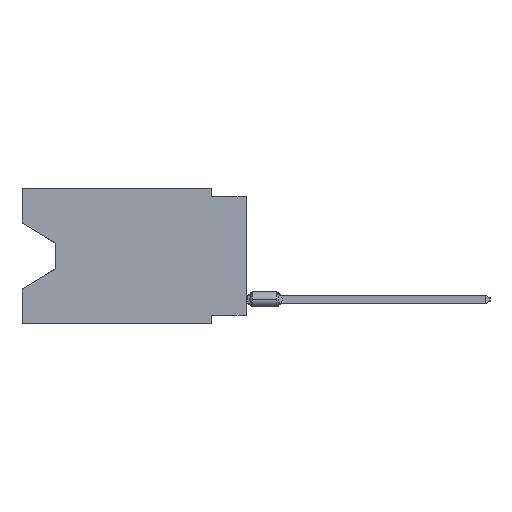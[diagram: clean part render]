
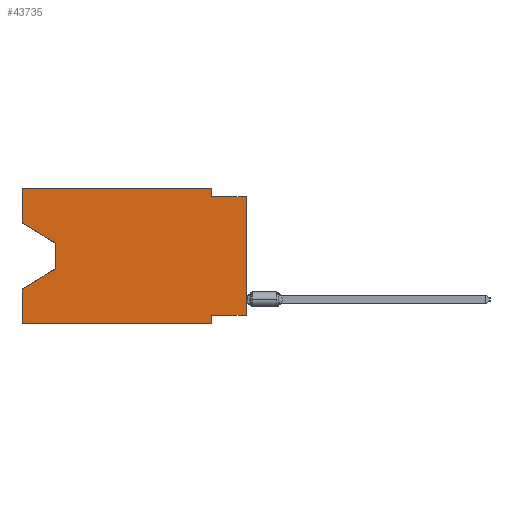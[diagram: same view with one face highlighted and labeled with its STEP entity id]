
A CAD part, left-side view. The second image highlights one B-rep face of the part: STEP entity #43735.
In plain terms, the highlighted planar face has unit normal (-1, 0, 0).
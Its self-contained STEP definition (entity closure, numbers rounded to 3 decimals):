
#249 = DIRECTION ( 'NONE',  ( 0., 0., 1. ) ) ;
#248 = VECTOR ( 'NONE', #21182, 1000. ) ;
#1300 = LINE ( 'NONE', #32505, #5962 ) ;
#2543 = LINE ( 'NONE', #37479, #35545 ) ;
#2876 = EDGE_CURVE ( 'NONE', #18927, #43641, #38914, .T. ) ;
#3427 = CARTESIAN_POINT ( 'NONE',  ( 0., 16.383, 0. ) ) ;
#4253 = VERTEX_POINT ( 'NONE', #3427 ) ;
#4367 = DIRECTION ( 'NONE',  ( 0., -1., 0. ) ) ;
#4447 = AXIS2_PLACEMENT_3D ( 'NONE', #50003, #10769, #25622 ) ;
#4461 = EDGE_CURVE ( 'NONE', #8686, #4253, #44630, .T. ) ;
#4482 = VERTEX_POINT ( 'NONE', #36317 ) ;
#5019 = ORIENTED_EDGE ( 'NONE', *, *, #14793, .F. ) ;
#5115 = CARTESIAN_POINT ( 'NONE',  ( 0., 0., 0. ) ) ;
#5689 = DIRECTION ( 'NONE',  ( 0., 0., 1. ) ) ;
#5962 = VECTOR ( 'NONE', #36523, 1000. ) ;
#7322 = DIRECTION ( 'NONE',  ( 0., 1., 0. ) ) ;
#8686 = VERTEX_POINT ( 'NONE', #26332 ) ;
#10237 = CARTESIAN_POINT ( 'NONE',  ( 0., 16.383, 0. ) ) ;
#10769 = DIRECTION ( 'NONE',  ( 1., 0., 0. ) ) ;
#11492 = EDGE_CURVE ( 'NONE', #17639, #19526, #2543, .T. ) ;
#11614 = LINE ( 'NONE', #29082, #48688 ) ;
#12200 = ORIENTED_EDGE ( 'NONE', *, *, #42566, .T. ) ;
#12966 = LINE ( 'NONE', #17823, #46207 ) ;
#13484 = EDGE_CURVE ( 'NONE', #18006, #26070, #25495, .T. ) ;
#13717 = CARTESIAN_POINT ( 'NONE',  ( 0., 16.383, 0. ) ) ;
#14038 = VECTOR ( 'NONE', #16965, 1000. ) ;
#14118 = EDGE_CURVE ( 'NONE', #42230, #4482, #30687, .T. ) ;
#14709 = CARTESIAN_POINT ( 'NONE',  ( 0., 13.97, -4.013 ) ) ;
#14792 = VECTOR ( 'NONE', #249, 1000. ) ;
#14793 = EDGE_CURVE ( 'NONE', #36934, #18006, #11614, .T. ) ;
#15066 = PLANE ( 'NONE',  #4447 ) ;
#15119 = DIRECTION ( 'NONE',  ( 0., 0., -1. ) ) ;
#15991 = DIRECTION ( 'NONE',  ( 0., -1., 0. ) ) ;
#16433 = CARTESIAN_POINT ( 'NONE',  ( 0., 16.383, -2.546 ) ) ;
#16965 = DIRECTION ( 'NONE',  ( 0., 0., -1. ) ) ;
#17252 = VECTOR ( 'NONE', #22578, 1000. ) ;
#17639 = VERTEX_POINT ( 'NONE', #36337 ) ;
#17823 = CARTESIAN_POINT ( 'NONE',  ( 0., 16.383, -9.906 ) ) ;
#18006 = VERTEX_POINT ( 'NONE', #36483 ) ;
#18927 = VERTEX_POINT ( 'NONE', #47924 ) ;
#19526 = VERTEX_POINT ( 'NONE', #38379 ) ;
#21182 = DIRECTION ( 'NONE',  ( 0., 0., -1. ) ) ;
#22578 = DIRECTION ( 'NONE',  ( 0., 0., 1. ) ) ;
#22694 = ORIENTED_EDGE ( 'NONE', *, *, #50847, .F. ) ;
#24102 = ORIENTED_EDGE ( 'NONE', *, *, #52577, .T. ) ;
#24240 = EDGE_LOOP ( 'NONE', ( #31747, #39656, #24102, #39378, #37430, #52296, #5019, #12200, #46076, #22694, #45834, #32801 ) ) ;
#24972 = VECTOR ( 'NONE', #33895, 1000. ) ;
#25495 = LINE ( 'NONE', #42964, #248 ) ;
#25622 = DIRECTION ( 'NONE',  ( 0., 0., -1. ) ) ;
#26070 = VERTEX_POINT ( 'NONE', #55886 ) ;
#26332 = CARTESIAN_POINT ( 'NONE',  ( 0., 16.383, -2.546 ) ) ;
#26478 = EDGE_CURVE ( 'NONE', #18927, #26070, #12966, .T. ) ;
#27667 = CARTESIAN_POINT ( 'NONE',  ( 0., 16.383, -7.36 ) ) ;
#28839 = LINE ( 'NONE', #36872, #29584 ) ;
#29082 = CARTESIAN_POINT ( 'NONE',  ( 0., 0., -9.271 ) ) ;
#29584 = VECTOR ( 'NONE', #15119, 1000. ) ;
#29905 = EDGE_CURVE ( 'NONE', #4253, #50880, #45455, .T. ) ;
#30687 = LINE ( 'NONE', #43884, #14038 ) ;
#31747 = ORIENTED_EDGE ( 'NONE', *, *, #49698, .T. ) ;
#32505 = CARTESIAN_POINT ( 'NONE',  ( 0., 13.97, -5.893 ) ) ;
#32801 = ORIENTED_EDGE ( 'NONE', *, *, #4461, .F. ) ;
#33895 = DIRECTION ( 'NONE',  ( 0., -0.855, -0.519 ) ) ;
#34062 = CARTESIAN_POINT ( 'NONE',  ( 0., 16.383, 0. ) ) ;
#35545 = VECTOR ( 'NONE', #15991, 1000. ) ;
#36317 = CARTESIAN_POINT ( 'NONE',  ( 0., 13.97, -5.893 ) ) ;
#36337 = CARTESIAN_POINT ( 'NONE',  ( 0., 2.54, -0.635 ) ) ;
#36483 = CARTESIAN_POINT ( 'NONE',  ( 0., 2.54, -9.271 ) ) ;
#36523 = DIRECTION ( 'NONE',  ( 0., 0.855, -0.519 ) ) ;
#36872 = CARTESIAN_POINT ( 'NONE',  ( 0., 2.54, 0. ) ) ;
#36934 = VERTEX_POINT ( 'NONE', #40720 ) ;
#37430 = ORIENTED_EDGE ( 'NONE', *, *, #26478, .T. ) ;
#37479 = CARTESIAN_POINT ( 'NONE',  ( 0., 0., -0.635 ) ) ;
#38379 = CARTESIAN_POINT ( 'NONE',  ( 0., 0., -0.635 ) ) ;
#38914 = LINE ( 'NONE', #34062, #14792 ) ;
#39378 = ORIENTED_EDGE ( 'NONE', *, *, #2876, .F. ) ;
#39582 = VECTOR ( 'NONE', #5689, 1000. ) ;
#39656 = ORIENTED_EDGE ( 'NONE', *, *, #14118, .T. ) ;
#40720 = CARTESIAN_POINT ( 'NONE',  ( 0., 0., -9.271 ) ) ;
#42230 = VERTEX_POINT ( 'NONE', #14709 ) ;
#42566 = EDGE_CURVE ( 'NONE', #36934, #19526, #44351, .T. ) ;
#42964 = CARTESIAN_POINT ( 'NONE',  ( 0., 2.54, -9.906 ) ) ;
#43594 = VECTOR ( 'NONE', #44596, 1000. ) ;
#43641 = VERTEX_POINT ( 'NONE', #27667 ) ;
#43735 = ADVANCED_FACE ( 'NONE', ( #54303 ), #15066, .F. ) ;
#43884 = CARTESIAN_POINT ( 'NONE',  ( 0., 13.97, -4.013 ) ) ;
#44351 = LINE ( 'NONE', #5115, #17252 ) ;
#44596 = DIRECTION ( 'NONE',  ( 0., -1., 0. ) ) ;
#44630 = LINE ( 'NONE', #13717, #39582 ) ;
#45455 = LINE ( 'NONE', #10237, #43594 ) ;
#45834 = ORIENTED_EDGE ( 'NONE', *, *, #29905, .F. ) ;
#46076 = ORIENTED_EDGE ( 'NONE', *, *, #11492, .F. ) ;
#46207 = VECTOR ( 'NONE', #4367, 1000. ) ;
#47924 = CARTESIAN_POINT ( 'NONE',  ( 0., 16.383, -9.906 ) ) ;
#48688 = VECTOR ( 'NONE', #7322, 1000. ) ;
#49698 = EDGE_CURVE ( 'NONE', #8686, #42230, #55683, .T. ) ;
#50003 = CARTESIAN_POINT ( 'NONE',  ( 0., 16.383, 0. ) ) ;
#50607 = CARTESIAN_POINT ( 'NONE',  ( 0., 2.54, 0. ) ) ;
#50847 = EDGE_CURVE ( 'NONE', #50880, #17639, #28839, .T. ) ;
#50880 = VERTEX_POINT ( 'NONE', #50607 ) ;
#52296 = ORIENTED_EDGE ( 'NONE', *, *, #13484, .F. ) ;
#52577 = EDGE_CURVE ( 'NONE', #4482, #43641, #1300, .T. ) ;
#54303 = FACE_OUTER_BOUND ( 'NONE', #24240, .T. ) ;
#55683 = LINE ( 'NONE', #16433, #24972 ) ;
#55886 = CARTESIAN_POINT ( 'NONE',  ( 0., 2.54, -9.906 ) ) ;
